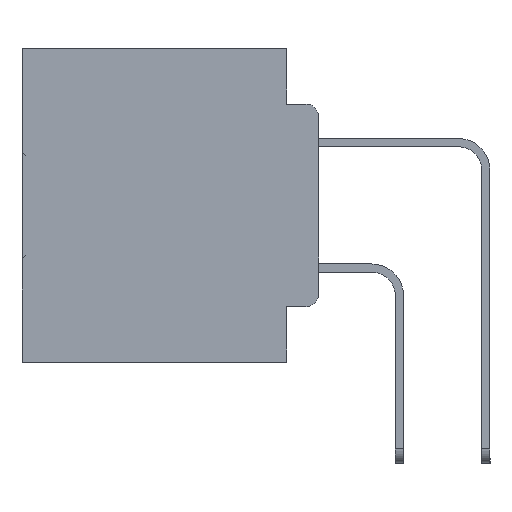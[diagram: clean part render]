
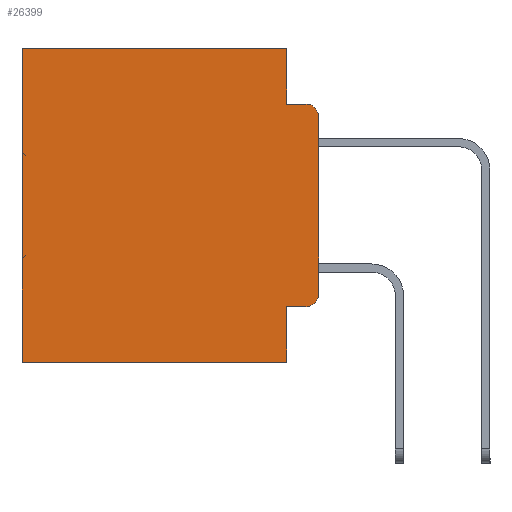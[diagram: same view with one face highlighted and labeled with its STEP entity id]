
A CAD part, left-side view. The second image highlights one B-rep face of the part: STEP entity #26399.
In plain terms, the highlighted planar face has unit normal (-1, 0, 0).
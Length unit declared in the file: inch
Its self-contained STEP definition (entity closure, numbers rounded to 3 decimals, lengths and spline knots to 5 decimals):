
#713 = LINE ( 'NONE', #4412, #14748 ) ;
#1077 = CARTESIAN_POINT ( 'NONE',  ( 0.298, 0., -0.3915 ) ) ;
#1628 = DIRECTION ( 'NONE',  ( 0., 0., -1. ) ) ;
#1907 = VECTOR ( 'NONE', #19287, 39.37008 ) ;
#1909 = DIRECTION ( 'NONE',  ( 0., 0., -1. ) ) ;
#2316 = EDGE_CURVE ( 'NONE', #26751, #25194, #18495, .T. ) ;
#2483 = CARTESIAN_POINT ( 'NONE',  ( 0.298, 0.02, -0.3915 ) ) ;
#2941 = EDGE_CURVE ( 'NONE', #5473, #18267, #10680, .T. ) ;
#3914 = VERTEX_POINT ( 'NONE', #22883 ) ;
#4120 = DIRECTION ( 'NONE',  ( 0., 0., -1. ) ) ;
#4412 = CARTESIAN_POINT ( 'NONE',  ( 0.298, 0.473, 0. ) ) ;
#5209 = CARTESIAN_POINT ( 'NONE',  ( 0.298, 0.051, 0. ) ) ;
#5263 = LINE ( 'NONE', #23568, #11868 ) ;
#5304 = DIRECTION ( 'NONE',  ( 0., 0., -1. ) ) ;
#5473 = VERTEX_POINT ( 'NONE', #20870 ) ;
#6298 = DIRECTION ( 'NONE',  ( 0., 1., 0. ) ) ;
#6662 = EDGE_CURVE ( 'NONE', #8531, #30304, #17833, .T. ) ;
#7472 = CIRCLE ( 'NONE', #17162, 0.02 ) ;
#7898 = LINE ( 'NONE', #12488, #29046 ) ;
#8531 = VERTEX_POINT ( 'NONE', #35409 ) ;
#10680 = LINE ( 'NONE', #14422, #31716 ) ;
#10709 = VERTEX_POINT ( 'NONE', #11096 ) ;
#11096 = CARTESIAN_POINT ( 'NONE',  ( 0.298, 0.051, -0.5 ) ) ;
#11868 = VECTOR ( 'NONE', #4120, 39.37008 ) ;
#12114 = CARTESIAN_POINT ( 'NONE',  ( 0.298, 0.051, -0.4115 ) ) ;
#12488 = CARTESIAN_POINT ( 'NONE',  ( 0.298, 0.051, -0.4115 ) ) ;
#12969 = CARTESIAN_POINT ( 'NONE',  ( 0.298, 0., 0. ) ) ;
#13179 = CARTESIAN_POINT ( 'NONE',  ( 0.298, 0.02, -0.1085 ) ) ;
#13734 = DIRECTION ( 'NONE',  ( 0., 0., -1. ) ) ;
#14268 = DIRECTION ( 'NONE',  ( 0., -1., 0. ) ) ;
#14422 = CARTESIAN_POINT ( 'NONE',  ( 0.298, 0.051, -0.0885 ) ) ;
#14748 = VECTOR ( 'NONE', #1628, 39.37008 ) ;
#15754 = VECTOR ( 'NONE', #13734, 39.37008 ) ;
#15788 = LINE ( 'NONE', #17357, #29550 ) ;
#15904 = DIRECTION ( 'NONE',  ( 0., 0., -1. ) ) ;
#15967 = EDGE_CURVE ( 'NONE', #26165, #8531, #7898, .T. ) ;
#16851 = ORIENTED_EDGE ( 'NONE', *, *, #6662, .T. ) ;
#17162 = AXIS2_PLACEMENT_3D ( 'NONE', #13179, #32363, #15904 ) ;
#17357 = CARTESIAN_POINT ( 'NONE',  ( 0.298, 0., -0.5 ) ) ;
#17808 = ORIENTED_EDGE ( 'NONE', *, *, #15967, .T. ) ;
#17833 = CIRCLE ( 'NONE', #26206, 0.02 ) ;
#18267 = VERTEX_POINT ( 'NONE', #18653 ) ;
#18495 = LINE ( 'NONE', #35347, #1907 ) ;
#18603 = DIRECTION ( 'NONE',  ( 1., 0., 0. ) ) ;
#18623 = ORIENTED_EDGE ( 'NONE', *, *, #25204, .F. ) ;
#18653 = CARTESIAN_POINT ( 'NONE',  ( 0.298, 0.02, -0.0885 ) ) ;
#18679 = DIRECTION ( 'NONE',  ( 0., 0., -1. ) ) ;
#18705 = ORIENTED_EDGE ( 'NONE', *, *, #24777, .F. ) ;
#19230 = ORIENTED_EDGE ( 'NONE', *, *, #29755, .T. ) ;
#19287 = DIRECTION ( 'NONE',  ( 0., 1., 0. ) ) ;
#19843 = ORIENTED_EDGE ( 'NONE', *, *, #2316, .T. ) ;
#20327 = ORIENTED_EDGE ( 'NONE', *, *, #27759, .F. ) ;
#20825 = ORIENTED_EDGE ( 'NONE', *, *, #2941, .F. ) ;
#20870 = CARTESIAN_POINT ( 'NONE',  ( 0.298, 0.051, -0.0885 ) ) ;
#21107 = ORIENTED_EDGE ( 'NONE', *, *, #35731, .T. ) ;
#21165 = EDGE_CURVE ( 'NONE', #3914, #30304, #5263, .T. ) ;
#21525 = ORIENTED_EDGE ( 'NONE', *, *, #21165, .F. ) ;
#21639 = EDGE_LOOP ( 'NONE', ( #21525, #21107, #20825, #20327, #19843, #19230, #18705, #18623, #17808, #16851 ) ) ;
#21977 = DIRECTION ( 'NONE',  ( -1., 0., 0. ) ) ;
#22883 = CARTESIAN_POINT ( 'NONE',  ( 0.298, 0., -0.1085 ) ) ;
#23089 = LINE ( 'NONE', #27403, #15754 ) ;
#23568 = CARTESIAN_POINT ( 'NONE',  ( 0.298, 0., 0. ) ) ;
#23900 = VERTEX_POINT ( 'NONE', #32289 ) ;
#24777 = EDGE_CURVE ( 'NONE', #10709, #23900, #15788, .T. ) ;
#25083 = LINE ( 'NONE', #29690, #32362 ) ;
#25194 = VERTEX_POINT ( 'NONE', #32794 ) ;
#25204 = EDGE_CURVE ( 'NONE', #26165, #10709, #23089, .T. ) ;
#26165 = VERTEX_POINT ( 'NONE', #12114 ) ;
#26206 = AXIS2_PLACEMENT_3D ( 'NONE', #2483, #21977, #5304 ) ;
#26399 = ADVANCED_FACE ( 'NONE', ( #26410 ), #34948, .F. ) ;
#26410 = FACE_OUTER_BOUND ( 'NONE', #21639, .T. ) ;
#26751 = VERTEX_POINT ( 'NONE', #5209 ) ;
#27403 = CARTESIAN_POINT ( 'NONE',  ( 0.298, 0.051, 0. ) ) ;
#27759 = EDGE_CURVE ( 'NONE', #26751, #5473, #25083, .T. ) ;
#29046 = VECTOR ( 'NONE', #31672, 39.37008 ) ;
#29550 = VECTOR ( 'NONE', #6298, 39.37008 ) ;
#29690 = CARTESIAN_POINT ( 'NONE',  ( 0.298, 0.051, 0. ) ) ;
#29755 = EDGE_CURVE ( 'NONE', #25194, #23900, #713, .T. ) ;
#30304 = VERTEX_POINT ( 'NONE', #1077 ) ;
#31672 = DIRECTION ( 'NONE',  ( 0., -1., 0. ) ) ;
#31716 = VECTOR ( 'NONE', #14268, 39.37008 ) ;
#32289 = CARTESIAN_POINT ( 'NONE',  ( 0.298, 0.473, -0.5 ) ) ;
#32362 = VECTOR ( 'NONE', #18679, 39.37008 ) ;
#32363 = DIRECTION ( 'NONE',  ( -1., 0., 0. ) ) ;
#32794 = CARTESIAN_POINT ( 'NONE',  ( 0.298, 0.473, 0. ) ) ;
#34867 = AXIS2_PLACEMENT_3D ( 'NONE', #12969, #18603, #1909 ) ;
#34948 = PLANE ( 'NONE',  #34867 ) ;
#35347 = CARTESIAN_POINT ( 'NONE',  ( 0.298, 0., 0. ) ) ;
#35409 = CARTESIAN_POINT ( 'NONE',  ( 0.298, 0.02, -0.4115 ) ) ;
#35731 = EDGE_CURVE ( 'NONE', #3914, #18267, #7472, .T. ) ;
